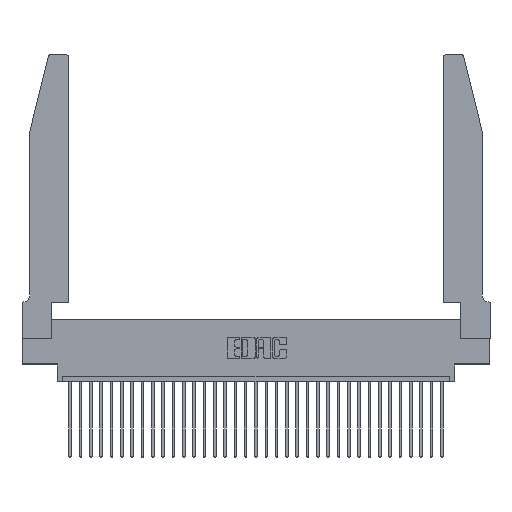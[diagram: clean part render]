
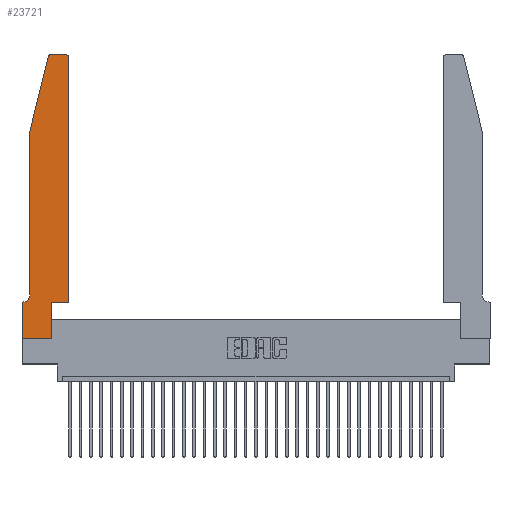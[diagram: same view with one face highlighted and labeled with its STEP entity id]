
A CAD part, top view. The second image highlights one B-rep face of the part: STEP entity #23721.
In plain terms, the highlighted planar face has unit normal (0, 0, 1).
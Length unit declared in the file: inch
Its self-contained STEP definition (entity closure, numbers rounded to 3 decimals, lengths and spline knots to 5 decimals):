
#9 = LINE ( 'NONE', #9889, #19776 ) ;
#350 = VERTEX_POINT ( 'NONE', #9494 ) ;
#464 = AXIS2_PLACEMENT_3D ( 'NONE', #7002, #17386, #17181 ) ;
#487 = CARTESIAN_POINT ( 'NONE',  ( 0.284, 2.72, 0.37 ) ) ;
#1124 = EDGE_CURVE ( 'NONE', #6356, #5477, #10476, .T. ) ;
#1620 = DIRECTION ( 'NONE',  ( -0.239, -0.971, 0. ) ) ;
#2166 = EDGE_CURVE ( 'NONE', #30757, #19641, #9, .T. ) ;
#2392 = ORIENTED_EDGE ( 'NONE', *, *, #11853, .T. ) ;
#3357 = EDGE_LOOP ( 'NONE', ( #16652, #23929, #18597, #17795, #4479, #27771, #12249, #2392, #12065, #14211, #31438, #17184 ) ) ;
#4220 = CIRCLE ( 'NONE', #6635, 0.07 ) ;
#4479 = ORIENTED_EDGE ( 'NONE', *, *, #15630, .T. ) ;
#5336 = EDGE_CURVE ( 'NONE', #350, #24928, #8685, .T. ) ;
#5477 = VERTEX_POINT ( 'NONE', #27523 ) ;
#5493 = EDGE_CURVE ( 'NONE', #19373, #350, #29679, .T. ) ;
#6356 = VERTEX_POINT ( 'NONE', #17952 ) ;
#6635 = AXIS2_PLACEMENT_3D ( 'NONE', #25809, #15641, #15528 ) ;
#6762 = VERTEX_POINT ( 'NONE', #14899 ) ;
#6825 = EDGE_CURVE ( 'NONE', #24301, #32355, #32031, .T. ) ;
#7002 = CARTESIAN_POINT ( 'NONE',  ( 0.4205, 2.72, 0.37 ) ) ;
#7340 = EDGE_CURVE ( 'NONE', #6762, #24301, #8938, .T. ) ;
#7483 = CARTESIAN_POINT ( 'NONE',  ( 0., 0., 0.37 ) ) ;
#7539 = LINE ( 'NONE', #13755, #19673 ) ;
#8136 = CARTESIAN_POINT ( 'NONE',  ( 0.4505, 2.72, 0.37 ) ) ;
#8516 = CARTESIAN_POINT ( 'NONE',  ( 0.284, 2.75, 0.37 ) ) ;
#8528 = LINE ( 'NONE', #7483, #18616 ) ;
#8685 = LINE ( 'NONE', #20970, #26880 ) ;
#8938 = LINE ( 'NONE', #11487, #32383 ) ;
#9011 = CIRCLE ( 'NONE', #18675, 0.03 ) ;
#9494 = CARTESIAN_POINT ( 'NONE',  ( 0., 0.35, 0.37 ) ) ;
#9889 = CARTESIAN_POINT ( 'NONE',  ( 0.2865, 0.35, 0.37 ) ) ;
#10395 = CARTESIAN_POINT ( 'NONE',  ( 0.0755, 2., 0.37 ) ) ;
#10476 = LINE ( 'NONE', #10395, #32718 ) ;
#10785 = EDGE_CURVE ( 'NONE', #26126, #17743, #9011, .T. ) ;
#10933 = VECTOR ( 'NONE', #1620, 39.37008 ) ;
#11487 = CARTESIAN_POINT ( 'NONE',  ( 0.4505, 0.35, 0.37 ) ) ;
#11754 = LINE ( 'NONE', #14349, #10933 ) ;
#11844 = DIRECTION ( 'NONE',  ( 1., 0., 0. ) ) ;
#11853 = EDGE_CURVE ( 'NONE', #24928, #30757, #8528, .T. ) ;
#12065 = ORIENTED_EDGE ( 'NONE', *, *, #2166, .T. ) ;
#12249 = ORIENTED_EDGE ( 'NONE', *, *, #5336, .T. ) ;
#12594 = PLANE ( 'NONE',  #25826 ) ;
#13214 = DIRECTION ( 'NONE',  ( 0., -1., 0. ) ) ;
#13755 = CARTESIAN_POINT ( 'NONE',  ( 0.2605, 2.75, 0.37 ) ) ;
#14211 = ORIENTED_EDGE ( 'NONE', *, *, #32258, .T. ) ;
#14349 = CARTESIAN_POINT ( 'NONE',  ( 0.0755, 2., 0.37 ) ) ;
#14397 = DIRECTION ( 'NONE',  ( -1., 0., 0. ) ) ;
#14868 = CARTESIAN_POINT ( 'NONE',  ( 0., 0.35, 0.37 ) ) ;
#14899 = CARTESIAN_POINT ( 'NONE',  ( 0.4505, 0.35, 0.37 ) ) ;
#15223 = CARTESIAN_POINT ( 'NONE',  ( 0.2865, 0.35, 0.37 ) ) ;
#15528 = DIRECTION ( 'NONE',  ( -1., 0., 0. ) ) ;
#15630 = EDGE_CURVE ( 'NONE', #5477, #19373, #4220, .T. ) ;
#15641 = DIRECTION ( 'NONE',  ( 0., 0., -1. ) ) ;
#16273 = CARTESIAN_POINT ( 'NONE',  ( 0.4505, 0.35, 0.37 ) ) ;
#16652 = ORIENTED_EDGE ( 'NONE', *, *, #26831, .T. ) ;
#17181 = DIRECTION ( 'NONE',  ( 1., 0., 0. ) ) ;
#17184 = ORIENTED_EDGE ( 'NONE', *, *, #6825, .T. ) ;
#17386 = DIRECTION ( 'NONE',  ( 0., 0., 1. ) ) ;
#17440 = CARTESIAN_POINT ( 'NONE',  ( 0.0755, 0.35, 0.37 ) ) ;
#17743 = VERTEX_POINT ( 'NONE', #27699 ) ;
#17795 = ORIENTED_EDGE ( 'NONE', *, *, #1124, .T. ) ;
#17952 = CARTESIAN_POINT ( 'NONE',  ( 0.0755, 2., 0.37 ) ) ;
#17987 = CARTESIAN_POINT ( 'NONE',  ( 0.0055, 0.35, 0.37 ) ) ;
#18597 = ORIENTED_EDGE ( 'NONE', *, *, #29385, .T. ) ;
#18616 = VECTOR ( 'NONE', #20478, 39.37008 ) ;
#18675 = AXIS2_PLACEMENT_3D ( 'NONE', #487, #28923, #23401 ) ;
#19373 = VERTEX_POINT ( 'NONE', #17987 ) ;
#19641 = VERTEX_POINT ( 'NONE', #15223 ) ;
#19673 = VECTOR ( 'NONE', #24521, 39.37008 ) ;
#19776 = VECTOR ( 'NONE', #26954, 39.37008 ) ;
#20175 = DIRECTION ( 'NONE',  ( 0., 0., 1. ) ) ;
#20478 = DIRECTION ( 'NONE',  ( 1., 0., 0. ) ) ;
#20970 = CARTESIAN_POINT ( 'NONE',  ( 0., 0., 0.37 ) ) ;
#21186 = LINE ( 'NONE', #16273, #29664 ) ;
#22269 = FACE_OUTER_BOUND ( 'NONE', #3357, .T. ) ;
#22434 = VECTOR ( 'NONE', #14397, 39.37008 ) ;
#23401 = DIRECTION ( 'NONE',  ( 1., 0., 0. ) ) ;
#23721 = ADVANCED_FACE ( 'NONE', ( #22269 ), #12594, .T. ) ;
#23929 = ORIENTED_EDGE ( 'NONE', *, *, #10785, .T. ) ;
#24301 = VERTEX_POINT ( 'NONE', #8136 ) ;
#24521 = DIRECTION ( 'NONE',  ( -1., 0., 0. ) ) ;
#24928 = VERTEX_POINT ( 'NONE', #26627 ) ;
#25438 = CARTESIAN_POINT ( 'NONE',  ( 0.2865, 0., 0.37 ) ) ;
#25809 = CARTESIAN_POINT ( 'NONE',  ( 0.0055, 0.42, 0.37 ) ) ;
#25826 = AXIS2_PLACEMENT_3D ( 'NONE', #14868, #20175, #32836 ) ;
#25827 = DIRECTION ( 'NONE',  ( 0., -1., 0. ) ) ;
#26126 = VERTEX_POINT ( 'NONE', #8516 ) ;
#26627 = CARTESIAN_POINT ( 'NONE',  ( 0., 0., 0.37 ) ) ;
#26831 = EDGE_CURVE ( 'NONE', #32355, #26126, #7539, .T. ) ;
#26880 = VECTOR ( 'NONE', #25827, 39.37008 ) ;
#26954 = DIRECTION ( 'NONE',  ( 0., 1., 0. ) ) ;
#26987 = DIRECTION ( 'NONE',  ( 0., 1., 0. ) ) ;
#27344 = CARTESIAN_POINT ( 'NONE',  ( 0.4205, 2.75, 0.37 ) ) ;
#27523 = CARTESIAN_POINT ( 'NONE',  ( 0.0755, 0.42, 0.37 ) ) ;
#27699 = CARTESIAN_POINT ( 'NONE',  ( 0.25487, 2.72718, 0.37 ) ) ;
#27771 = ORIENTED_EDGE ( 'NONE', *, *, #5493, .T. ) ;
#28923 = DIRECTION ( 'NONE',  ( 0., 0., 1. ) ) ;
#29385 = EDGE_CURVE ( 'NONE', #17743, #6356, #11754, .T. ) ;
#29664 = VECTOR ( 'NONE', #11844, 39.37008 ) ;
#29679 = LINE ( 'NONE', #17440, #22434 ) ;
#30757 = VERTEX_POINT ( 'NONE', #25438 ) ;
#31438 = ORIENTED_EDGE ( 'NONE', *, *, #7340, .T. ) ;
#32031 = CIRCLE ( 'NONE', #464, 0.03 ) ;
#32258 = EDGE_CURVE ( 'NONE', #19641, #6762, #21186, .T. ) ;
#32355 = VERTEX_POINT ( 'NONE', #27344 ) ;
#32383 = VECTOR ( 'NONE', #26987, 39.37008 ) ;
#32718 = VECTOR ( 'NONE', #13214, 39.37008 ) ;
#32836 = DIRECTION ( 'NONE',  ( 1., 0., 0. ) ) ;
